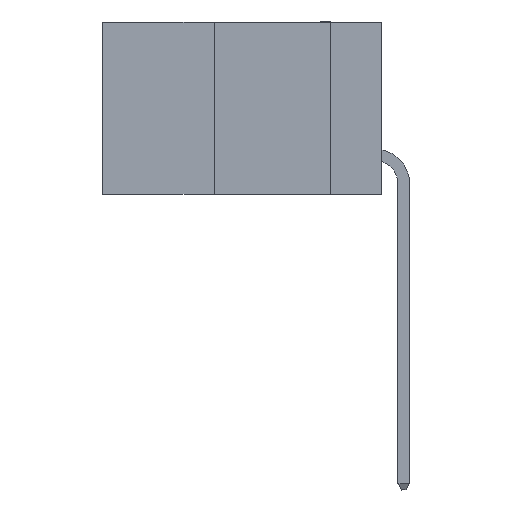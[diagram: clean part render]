
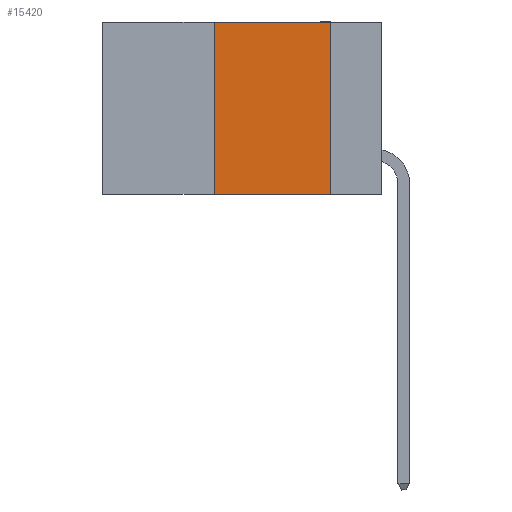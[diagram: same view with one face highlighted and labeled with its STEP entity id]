
A CAD part, left-side view. The second image highlights one B-rep face of the part: STEP entity #15420.
In plain terms, the highlighted planar face has unit normal (-1, 0, 0).
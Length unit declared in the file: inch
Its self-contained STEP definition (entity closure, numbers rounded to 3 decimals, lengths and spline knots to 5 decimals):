
#1459 = ORIENTED_EDGE ( 'NONE', *, *, #23662, .F. ) ;
#2089 = CARTESIAN_POINT ( 'NONE',  ( 0., 0.11, 0. ) ) ;
#2745 = DIRECTION ( 'NONE',  ( 0., 0., -1. ) ) ;
#3547 = VERTEX_POINT ( 'NONE', #9665 ) ;
#4163 = DIRECTION ( 'NONE',  ( 0., 0., 1. ) ) ;
#4871 = VERTEX_POINT ( 'NONE', #6736 ) ;
#6736 = CARTESIAN_POINT ( 'NONE',  ( 0., 0.36, -0.37 ) ) ;
#6900 = VERTEX_POINT ( 'NONE', #2089 ) ;
#7752 = EDGE_CURVE ( 'NONE', #3547, #6900, #9162, .T. ) ;
#8407 = VERTEX_POINT ( 'NONE', #11163 ) ;
#9162 = LINE ( 'NONE', #14727, #15490 ) ;
#9171 = LINE ( 'NONE', #17660, #23438 ) ;
#9312 = DIRECTION ( 'NONE',  ( 1., 0., 0. ) ) ;
#9665 = CARTESIAN_POINT ( 'NONE',  ( 0., 0.36, 0. ) ) ;
#11163 = CARTESIAN_POINT ( 'NONE',  ( 0., 0.11, -0.37 ) ) ;
#13245 = VECTOR ( 'NONE', #27239, 39.37008 ) ;
#13289 = EDGE_LOOP ( 'NONE', ( #25231, #16863, #1459, #22394 ) ) ;
#13342 = VECTOR ( 'NONE', #25313, 39.37008 ) ;
#14029 = CARTESIAN_POINT ( 'NONE',  ( 0., 0.6, 0. ) ) ;
#14727 = CARTESIAN_POINT ( 'NONE',  ( 0., 0.6, 0. ) ) ;
#15420 = ADVANCED_FACE ( 'NONE', ( #27155 ), #19467, .F. ) ;
#15490 = VECTOR ( 'NONE', #15588, 39.37008 ) ;
#15588 = DIRECTION ( 'NONE',  ( 0., -1., 0. ) ) ;
#16863 = ORIENTED_EDGE ( 'NONE', *, *, #7752, .F. ) ;
#17660 = CARTESIAN_POINT ( 'NONE',  ( 0., 0.36, 0. ) ) ;
#18507 = CARTESIAN_POINT ( 'NONE',  ( 0., 0.11, 0. ) ) ;
#18797 = EDGE_CURVE ( 'NONE', #6900, #8407, #23386, .T. ) ;
#19467 = PLANE ( 'NONE',  #23767 ) ;
#21024 = EDGE_CURVE ( 'NONE', #4871, #8407, #25729, .T. ) ;
#22394 = ORIENTED_EDGE ( 'NONE', *, *, #21024, .T. ) ;
#23386 = LINE ( 'NONE', #18507, #13342 ) ;
#23438 = VECTOR ( 'NONE', #4163, 39.37008 ) ;
#23662 = EDGE_CURVE ( 'NONE', #4871, #3547, #9171, .T. ) ;
#23767 = AXIS2_PLACEMENT_3D ( 'NONE', #14029, #9312, #2745 ) ;
#25231 = ORIENTED_EDGE ( 'NONE', *, *, #18797, .F. ) ;
#25313 = DIRECTION ( 'NONE',  ( 0., 0., -1. ) ) ;
#25729 = LINE ( 'NONE', #27047, #13245 ) ;
#27047 = CARTESIAN_POINT ( 'NONE',  ( 0., 0.6, -0.37 ) ) ;
#27155 = FACE_OUTER_BOUND ( 'NONE', #13289, .T. ) ;
#27239 = DIRECTION ( 'NONE',  ( 0., -1., 0. ) ) ;
